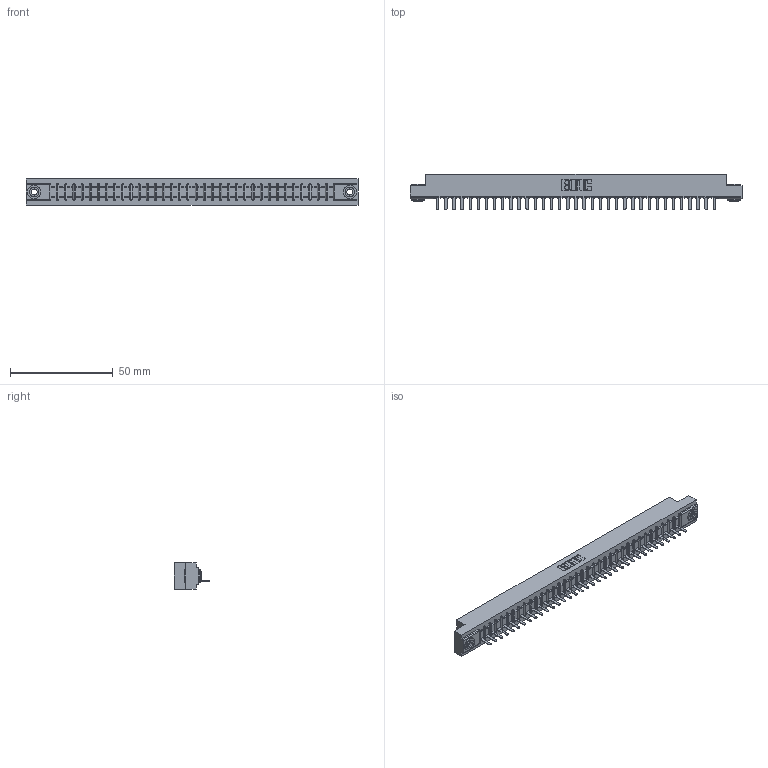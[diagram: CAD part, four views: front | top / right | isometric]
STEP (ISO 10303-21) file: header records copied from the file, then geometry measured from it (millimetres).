
FILE_DESCRIPTION (( 'STEP AP203' ), '1' );
FILE_NAME ('307-035-521-103.STEP', '2019-09-05T07:03:31', ( '' ), ( '' ), 'SwSTEP 2.0', 'SolidWorks 2016', '' );
FILE_SCHEMA (( 'CONFIG_CONTROL_DESIGN' ));
Length unit declared in the file: inch
Products named in the file (4): 307-035-521-103; 307 Part_.156 Dia Mounting Holes; 307-290-002_521; 345-250-002_345-250-002-102
Assembly tree (38 placements, depth 2):
  307-035-521-103
    307 Part_.156 Dia Mounting Holes
    307-290-002_521  x35
    345-250-002_345-250-002-102  x2
Bounding box: 161.7 x 17.42 x 12.7 mm (x, y, z)
Volume: 17254.7 mm3; surface area: 21797.2 mm2
Topology: 38 solids, 38 shells, 2796 faces, 8555 edges, 5602 vertices
Faces by surface type: plane 1669, cylinder 1047, sphere 72, cone 8
Entity records: 32651 total; most frequent: CARTESIAN_POINT 5485, ORIENTED_EDGE 5466, DIRECTION 5347, EDGE_CURVE 2733, VECTOR 2083, LINE 2083, VERTEX_POINT 1770, AXIS2_PLACEMENT_3D 1632
